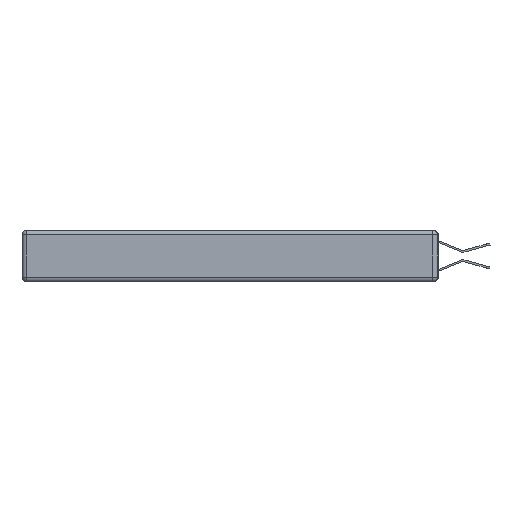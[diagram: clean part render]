
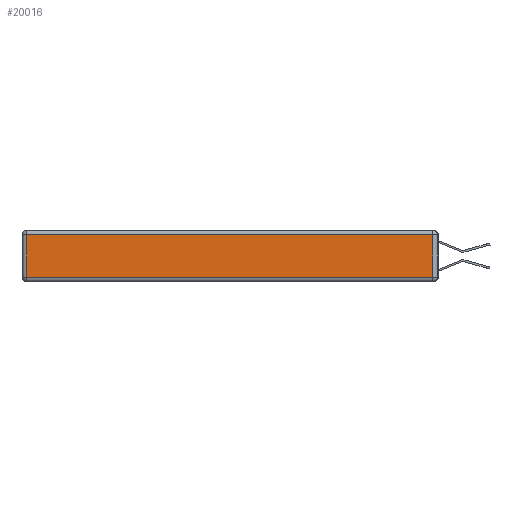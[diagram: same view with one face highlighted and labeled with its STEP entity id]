
A CAD part, left-side view. The second image highlights one B-rep face of the part: STEP entity #20016.
In plain terms, the highlighted planar face has unit normal (-1, 0, 0).
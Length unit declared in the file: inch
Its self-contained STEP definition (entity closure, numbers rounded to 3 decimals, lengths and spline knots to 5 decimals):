
#438 = ORIENTED_EDGE ( 'NONE', *, *, #24551, .T. ) ;
#612 = LINE ( 'NONE', #18505, #21692 ) ;
#804 = CARTESIAN_POINT ( 'NONE',  ( 0., 2.72, -0.313 ) ) ;
#1040 = DIRECTION ( 'NONE',  ( -1., 0., 0. ) ) ;
#1165 = FACE_OUTER_BOUND ( 'NONE', #25400, .T. ) ;
#2038 = VERTEX_POINT ( 'NONE', #4183 ) ;
#2174 = DIRECTION ( 'NONE',  ( 0., 0., 1. ) ) ;
#2426 = CARTESIAN_POINT ( 'NONE',  ( 0., 0.03, -0.343 ) ) ;
#3586 = CARTESIAN_POINT ( 'NONE',  ( 0., 0.03, -0.03 ) ) ;
#3611 = VERTEX_POINT ( 'NONE', #804 ) ;
#4183 = CARTESIAN_POINT ( 'NONE',  ( 0., 2.72, -0.03 ) ) ;
#6489 = LINE ( 'NONE', #2426, #14463 ) ;
#6554 = ORIENTED_EDGE ( 'NONE', *, *, #21077, .T. ) ;
#7208 = PLANE ( 'NONE',  #24249 ) ;
#7290 = EDGE_CURVE ( 'NONE', #11444, #2038, #612, .T. ) ;
#8989 = LINE ( 'NONE', #10428, #15675 ) ;
#10386 = DIRECTION ( 'NONE',  ( 0., 1., 0. ) ) ;
#10428 = CARTESIAN_POINT ( 'NONE',  ( 0., 0., -0.313 ) ) ;
#10806 = DIRECTION ( 'NONE',  ( 0., 0., -1. ) ) ;
#11027 = ORIENTED_EDGE ( 'NONE', *, *, #7290, .T. ) ;
#11444 = VERTEX_POINT ( 'NONE', #3586 ) ;
#14463 = VECTOR ( 'NONE', #2174, 39.37008 ) ;
#15074 = CARTESIAN_POINT ( 'NONE',  ( 0., 0., -0.343 ) ) ;
#15112 = CARTESIAN_POINT ( 'NONE',  ( 0., 2.72, -0.343 ) ) ;
#15675 = VECTOR ( 'NONE', #24609, 39.37008 ) ;
#16141 = VECTOR ( 'NONE', #10806, 39.37008 ) ;
#16772 = LINE ( 'NONE', #15112, #16141 ) ;
#17400 = EDGE_CURVE ( 'NONE', #3611, #20600, #8989, .T. ) ;
#18505 = CARTESIAN_POINT ( 'NONE',  ( 0., 2.75, -0.03 ) ) ;
#19497 = DIRECTION ( 'NONE',  ( 0., 0., 1. ) ) ;
#20016 = ADVANCED_FACE ( 'NONE', ( #1165 ), #7208, .T. ) ;
#20103 = ORIENTED_EDGE ( 'NONE', *, *, #17400, .T. ) ;
#20600 = VERTEX_POINT ( 'NONE', #23676 ) ;
#21077 = EDGE_CURVE ( 'NONE', #2038, #3611, #16772, .T. ) ;
#21692 = VECTOR ( 'NONE', #10386, 39.37008 ) ;
#23676 = CARTESIAN_POINT ( 'NONE',  ( 0., 0.03, -0.313 ) ) ;
#24249 = AXIS2_PLACEMENT_3D ( 'NONE', #15074, #1040, #19497 ) ;
#24551 = EDGE_CURVE ( 'NONE', #20600, #11444, #6489, .T. ) ;
#24609 = DIRECTION ( 'NONE',  ( 0., -1., 0. ) ) ;
#25400 = EDGE_LOOP ( 'NONE', ( #20103, #438, #11027, #6554 ) ) ;
